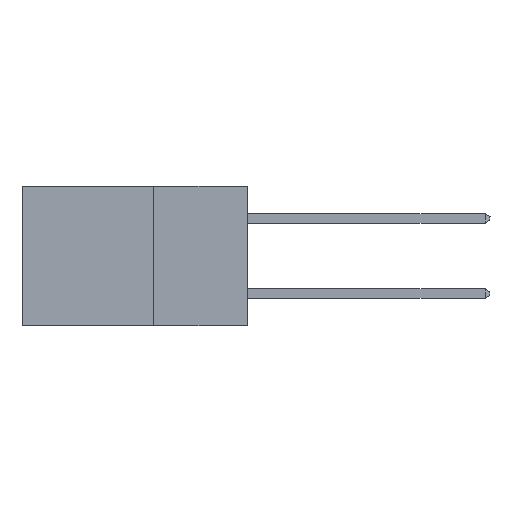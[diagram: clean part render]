
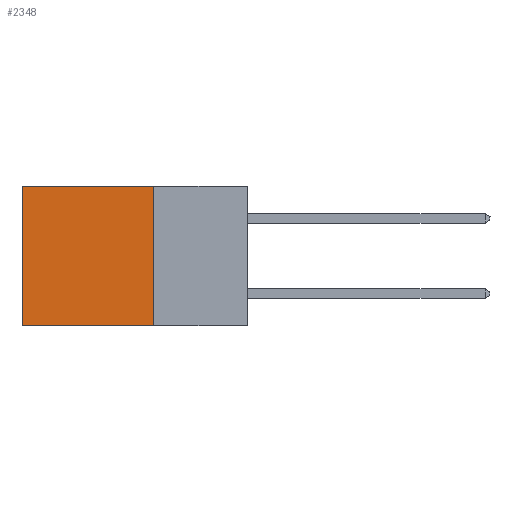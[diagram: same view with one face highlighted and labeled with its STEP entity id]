
A CAD part, left-side view. The second image highlights one B-rep face of the part: STEP entity #2348.
In plain terms, the highlighted planar face has unit normal (-1, 0, 0).
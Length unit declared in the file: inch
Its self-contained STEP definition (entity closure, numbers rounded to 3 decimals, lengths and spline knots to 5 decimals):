
#769 = VERTEX_POINT ( 'NONE', #16936 ) ;
#1448 = LINE ( 'NONE', #13258, #2863 ) ;
#1732 = CARTESIAN_POINT ( 'NONE',  ( 0.2615, 0.25, -0.37 ) ) ;
#2348 = ADVANCED_FACE ( 'NONE', ( #18117 ), #8209, .F. ) ;
#2409 = VERTEX_POINT ( 'NONE', #18001 ) ;
#2580 = ORIENTED_EDGE ( 'NONE', *, *, #18733, .F. ) ;
#2863 = VECTOR ( 'NONE', #13142, 39.37008 ) ;
#3231 = DIRECTION ( 'NONE',  ( 0., 0., -1. ) ) ;
#3588 = AXIS2_PLACEMENT_3D ( 'NONE', #1732, #16475, #6372 ) ;
#4411 = CARTESIAN_POINT ( 'NONE',  ( 0.2615, 0.25, -0.37 ) ) ;
#5000 = LINE ( 'NONE', #7897, #17694 ) ;
#6060 = ORIENTED_EDGE ( 'NONE', *, *, #14085, .F. ) ;
#6372 = DIRECTION ( 'NONE',  ( 0., 0., -1. ) ) ;
#6423 = VECTOR ( 'NONE', #9711, 39.37008 ) ;
#6678 = LINE ( 'NONE', #16547, #6423 ) ;
#7111 = CARTESIAN_POINT ( 'NONE',  ( 0.2615, 0.6, 0. ) ) ;
#7396 = EDGE_CURVE ( 'NONE', #10281, #2409, #5000, .T. ) ;
#7897 = CARTESIAN_POINT ( 'NONE',  ( 0.2615, 0.6, -0.37 ) ) ;
#8209 = PLANE ( 'NONE',  #3588 ) ;
#9061 = EDGE_CURVE ( 'NONE', #18494, #10281, #1448, .T. ) ;
#9711 = DIRECTION ( 'NONE',  ( 0., 1., 0. ) ) ;
#10281 = VERTEX_POINT ( 'NONE', #7111 ) ;
#13142 = DIRECTION ( 'NONE',  ( 0., 1., 0. ) ) ;
#13258 = CARTESIAN_POINT ( 'NONE',  ( 0.2615, 0.25, 0. ) ) ;
#14085 = EDGE_CURVE ( 'NONE', #769, #2409, #6678, .T. ) ;
#16079 = EDGE_LOOP ( 'NONE', ( #21171, #6060, #2580, #20591 ) ) ;
#16475 = DIRECTION ( 'NONE',  ( 1., 0., 0. ) ) ;
#16547 = CARTESIAN_POINT ( 'NONE',  ( 0.2615, 0.25, -0.37 ) ) ;
#16793 = CARTESIAN_POINT ( 'NONE',  ( 0.2615, 0.25, 0. ) ) ;
#16936 = CARTESIAN_POINT ( 'NONE',  ( 0.2615, 0.25, -0.37 ) ) ;
#17694 = VECTOR ( 'NONE', #17898, 39.37008 ) ;
#17898 = DIRECTION ( 'NONE',  ( 0., 0., -1. ) ) ;
#17956 = VECTOR ( 'NONE', #3231, 39.37008 ) ;
#18001 = CARTESIAN_POINT ( 'NONE',  ( 0.2615, 0.6, -0.37 ) ) ;
#18117 = FACE_OUTER_BOUND ( 'NONE', #16079, .T. ) ;
#18494 = VERTEX_POINT ( 'NONE', #16793 ) ;
#18733 = EDGE_CURVE ( 'NONE', #18494, #769, #20996, .T. ) ;
#20591 = ORIENTED_EDGE ( 'NONE', *, *, #9061, .T. ) ;
#20996 = LINE ( 'NONE', #4411, #17956 ) ;
#21171 = ORIENTED_EDGE ( 'NONE', *, *, #7396, .T. ) ;
